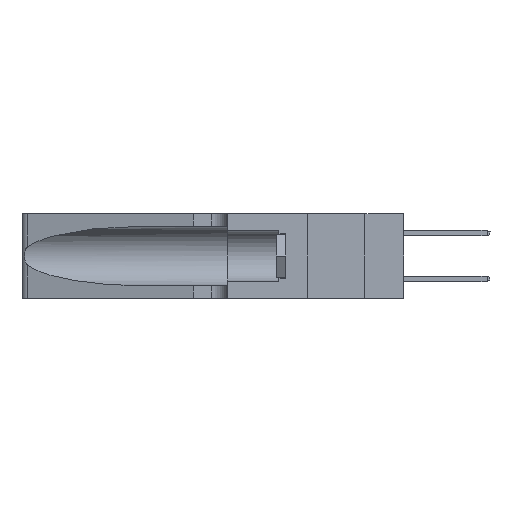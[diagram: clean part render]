
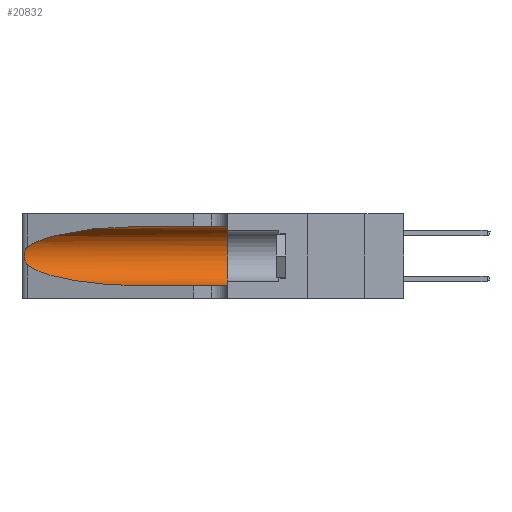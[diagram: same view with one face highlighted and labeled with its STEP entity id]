
A CAD part, left-side view. The second image highlights one B-rep face of the part: STEP entity #20832.
In plain terms, the highlighted cylindrical face has radius 3.308 mm (diameter 6.617 mm), a partial arc.
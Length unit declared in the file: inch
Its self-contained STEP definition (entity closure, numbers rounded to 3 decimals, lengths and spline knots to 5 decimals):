
#1591 = CIRCLE ( 'NONE', #5752, 0.13025 ) ;
#1693 = CARTESIAN_POINT ( 'NONE',  ( 0.26075, 1.23896, 0.178 ) ) ;
#2007 = EDGE_CURVE ( 'NONE', #5773, #6701, #6177, .T. ) ;
#2186 =( BOUNDED_CURVE ( )  B_SPLINE_CURVE ( 3, ( #12332, #19342, #8509, #3147 ),
 .UNSPECIFIED., .F., .T. ) 
 B_SPLINE_CURVE_WITH_KNOTS ( ( 4, 4 ),
 ( 1.5708, 2.84003 ),
 .UNSPECIFIED. ) 
 CURVE ( )  GEOMETRIC_REPRESENTATION_ITEM ( )  RATIONAL_B_SPLINE_CURVE ( ( 1., 0.87, 0.87, 1. ) ) 
 REPRESENTATION_ITEM ( '' )  );
#2694 = ORIENTED_EDGE ( 'NONE', *, *, #19662, .T. ) ;
#3147 = CARTESIAN_POINT ( 'NONE',  ( 0.25487, 1.22718, 0.22369 ) ) ;
#3292 = CARTESIAN_POINT ( 'NONE',  ( 0.25639, 1.23184, 0.21858 ) ) ;
#3820 = CARTESIAN_POINT ( 'NONE',  ( 0.25789, 1.23486, 0.15765 ) ) ;
#4015 = ORIENTED_EDGE ( 'NONE', *, *, #18768, .T. ) ;
#4666 = ORIENTED_EDGE ( 'NONE', *, *, #19839, .T. ) ;
#4988 = DIRECTION ( 'NONE',  ( 0., -1., 0. ) ) ;
#5752 = AXIS2_PLACEMENT_3D ( 'NONE', #15495, #12003, #8121 ) ;
#5773 = VERTEX_POINT ( 'NONE', #9730 ) ;
#5875 = CARTESIAN_POINT ( 'NONE',  ( 0.1305, 0.35, 0.31525 ) ) ;
#6177 =( BOUNDED_CURVE ( )  B_SPLINE_CURVE ( 3, ( #13710, #7910, #22688, #19113 ),
 .UNSPECIFIED., .F., .F. ) 
 B_SPLINE_CURVE_WITH_KNOTS ( ( 4, 4 ),
 ( 3.44316, 4.71239 ),
 .UNSPECIFIED. ) 
 CURVE ( )  GEOMETRIC_REPRESENTATION_ITEM ( )  RATIONAL_B_SPLINE_CURVE ( ( 1., 0.87, 0.87, 1. ) ) 
 REPRESENTATION_ITEM ( '' )  );
#6227 = DIRECTION ( 'NONE',  ( 0., -1., 0. ) ) ;
#6319 = VECTOR ( 'NONE', #6227, 39.37008 ) ;
#6701 = VERTEX_POINT ( 'NONE', #11927 ) ;
#7173 = LINE ( 'NONE', #15269, #6319 ) ;
#7910 = CARTESIAN_POINT ( 'NONE',  ( 0.2373, 1.15595, 0.08982 ) ) ;
#8087 = CARTESIAN_POINT ( 'NONE',  ( 0.1305, 0.72297, 0.31525 ) ) ;
#8121 = DIRECTION ( 'NONE',  ( 0., 0., 1. ) ) ;
#8152 = CARTESIAN_POINT ( 'NONE',  ( 0.1305, 1.61858, 0.185 ) ) ;
#8509 = CARTESIAN_POINT ( 'NONE',  ( 0.2373, 1.15595, 0.28018 ) ) ;
#8723 = CARTESIAN_POINT ( 'NONE',  ( 0.25787, 1.23484, 0.2124 ) ) ;
#8800 = CARTESIAN_POINT ( 'NONE',  ( 0.25487, 1.22718, 0.22369 ) ) ;
#8959 = CARTESIAN_POINT ( 'NONE',  ( 0.26018, 1.23835, 0.19895 ) ) ;
#9277 = LINE ( 'NONE', #16037, #11579 ) ;
#9605 = VERTEX_POINT ( 'NONE', #9999 ) ;
#9730 = CARTESIAN_POINT ( 'NONE',  ( 0.25487, 1.22718, 0.14631 ) ) ;
#9999 = CARTESIAN_POINT ( 'NONE',  ( 0.1305, 0.35, 0.05475 ) ) ;
#10898 = ORIENTED_EDGE ( 'NONE', *, *, #2007, .T. ) ;
#11040 = ORIENTED_EDGE ( 'NONE', *, *, #18665, .F. ) ;
#11096 = B_SPLINE_CURVE_WITH_KNOTS ( 'NONE', 3,
 ( #8800, #17962, #3292, #8723, #21547, #8959, #23508, #1693, #14452, #16437, #3820, #14680, #20175, #18348 ),
 .UNSPECIFIED., .F., .F.,
 ( 4, 2, 2, 2, 2, 2, 4 ),
 ( 0., 0.00027, 0.00053, 0.00107, 0.0016, 0.00187, 0.00214 ),
 .UNSPECIFIED. ) ;
#11579 = VECTOR ( 'NONE', #4988, 39.37008 ) ;
#11927 = CARTESIAN_POINT ( 'NONE',  ( 0.1305, 0.72297, 0.05475 ) ) ;
#12003 = DIRECTION ( 'NONE',  ( 0., 1., 0. ) ) ;
#12332 = CARTESIAN_POINT ( 'NONE',  ( 0.1305, 0.72297, 0.31525 ) ) ;
#12380 = AXIS2_PLACEMENT_3D ( 'NONE', #8152, #19126, #20885 ) ;
#13710 = CARTESIAN_POINT ( 'NONE',  ( 0.25487, 1.22718, 0.14631 ) ) ;
#14129 = CARTESIAN_POINT ( 'NONE',  ( 0.25487, 1.22718, 0.22369 ) ) ;
#14452 = CARTESIAN_POINT ( 'NONE',  ( 0.26017, 1.23833, 0.17102 ) ) ;
#14594 = EDGE_CURVE ( 'NONE', #22543, #19354, #7173, .T. ) ;
#14680 = CARTESIAN_POINT ( 'NONE',  ( 0.25639, 1.23186, 0.15144 ) ) ;
#15269 = CARTESIAN_POINT ( 'NONE',  ( 0.1305, 1.61858, 0.31525 ) ) ;
#15495 = CARTESIAN_POINT ( 'NONE',  ( 0.1305, 0.35, 0.185 ) ) ;
#15503 = ORIENTED_EDGE ( 'NONE', *, *, #14594, .F. ) ;
#16037 = CARTESIAN_POINT ( 'NONE',  ( 0.1305, 1.61858, 0.05475 ) ) ;
#16437 = CARTESIAN_POINT ( 'NONE',  ( 0.25856, 1.23593, 0.16098 ) ) ;
#17623 = VERTEX_POINT ( 'NONE', #14129 ) ;
#17962 = CARTESIAN_POINT ( 'NONE',  ( 0.25555, 1.22994, 0.2215 ) ) ;
#18348 = CARTESIAN_POINT ( 'NONE',  ( 0.25487, 1.22718, 0.14631 ) ) ;
#18665 = EDGE_CURVE ( 'NONE', #19354, #9605, #1591, .T. ) ;
#18768 = EDGE_CURVE ( 'NONE', #6701, #9605, #9277, .T. ) ;
#19113 = CARTESIAN_POINT ( 'NONE',  ( 0.1305, 0.72297, 0.05475 ) ) ;
#19126 = DIRECTION ( 'NONE',  ( 0., -1., 0. ) ) ;
#19342 = CARTESIAN_POINT ( 'NONE',  ( 0.18966, 0.96281, 0.31525 ) ) ;
#19354 = VERTEX_POINT ( 'NONE', #5875 ) ;
#19662 = EDGE_CURVE ( 'NONE', #22543, #17623, #2186, .T. ) ;
#19839 = EDGE_CURVE ( 'NONE', #17623, #5773, #11096, .T. ) ;
#20175 = CARTESIAN_POINT ( 'NONE',  ( 0.25555, 1.22993, 0.14849 ) ) ;
#20286 = EDGE_LOOP ( 'NONE', ( #2694, #4666, #10898, #4015, #11040, #15503 ) ) ;
#20832 = ADVANCED_FACE ( 'NONE', ( #21724 ), #23143, .F. ) ;
#20885 = DIRECTION ( 'NONE',  ( 0., 0., -1. ) ) ;
#21547 = CARTESIAN_POINT ( 'NONE',  ( 0.25854, 1.2359, 0.20912 ) ) ;
#21724 = FACE_OUTER_BOUND ( 'NONE', #20286, .T. ) ;
#22543 = VERTEX_POINT ( 'NONE', #8087 ) ;
#22688 = CARTESIAN_POINT ( 'NONE',  ( 0.18966, 0.96281, 0.05475 ) ) ;
#23143 = CYLINDRICAL_SURFACE ( 'NONE', #12380, 0.13025 ) ;
#23508 = CARTESIAN_POINT ( 'NONE',  ( 0.26075, 1.23896, 0.19203 ) ) ;
